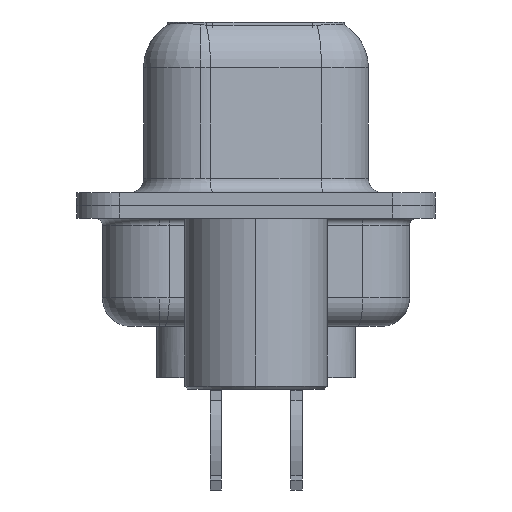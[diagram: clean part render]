
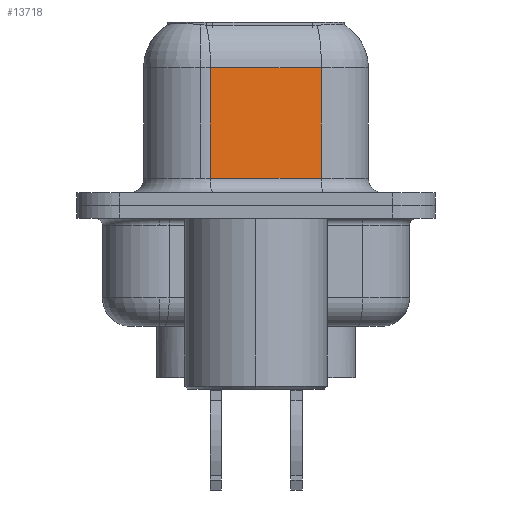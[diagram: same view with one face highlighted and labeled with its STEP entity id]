
A CAD part, left-side view. The second image highlights one B-rep face of the part: STEP entity #13718.
In plain terms, the highlighted planar face has unit normal (-0.985, -0.174, 0).
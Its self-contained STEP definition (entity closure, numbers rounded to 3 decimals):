
#380 = EDGE_CURVE ( 'NONE', #8218, #2512, #3110, .T. ) ;
#396 = CARTESIAN_POINT ( 'NONE',  ( 4.375, 1.603, 6.6 ) ) ;
#595 = DIRECTION ( 'NONE',  ( 0., 0., -1. ) ) ;
#1016 = VECTOR ( 'NONE', #13567, 1000. ) ;
#1240 = CARTESIAN_POINT ( 'NONE',  ( 5.063, -2.297, 6.6 ) ) ;
#1631 = LINE ( 'NONE', #396, #9218 ) ;
#1772 = DIRECTION ( 'NONE',  ( 0., 0., -1. ) ) ;
#2512 = VERTEX_POINT ( 'NONE', #15693 ) ;
#2651 = CARTESIAN_POINT ( 'NONE',  ( 5.063, -2.297, 4.85 ) ) ;
#3096 = DIRECTION ( 'NONE',  ( 0.985, 0.174, 0. ) ) ;
#3110 = LINE ( 'NONE', #4564, #11971 ) ;
#4564 = CARTESIAN_POINT ( 'NONE',  ( 5.063, -2.297, 6.6 ) ) ;
#5290 = LINE ( 'NONE', #16024, #9654 ) ;
#7243 = LINE ( 'NONE', #8904, #1016 ) ;
#8218 = VERTEX_POINT ( 'NONE', #2651 ) ;
#8488 = CARTESIAN_POINT ( 'NONE',  ( 4.375, 1.603, 0.95 ) ) ;
#8558 = VERTEX_POINT ( 'NONE', #8488 ) ;
#8904 = CARTESIAN_POINT ( 'NONE',  ( 5.063, -2.297, 4.85 ) ) ;
#9218 = VECTOR ( 'NONE', #595, 1000. ) ;
#9340 = EDGE_CURVE ( 'NONE', #17225, #8558, #1631, .T. ) ;
#9654 = VECTOR ( 'NONE', #11631, 1000. ) ;
#10092 = AXIS2_PLACEMENT_3D ( 'NONE', #1240, #3096, #15787 ) ;
#10482 = EDGE_LOOP ( 'NONE', ( #16739, #15724, #15220, #19773 ) ) ;
#11631 = DIRECTION ( 'NONE',  ( 0.174, -0.985, 0. ) ) ;
#11931 = CARTESIAN_POINT ( 'NONE',  ( 4.375, 1.603, 4.85 ) ) ;
#11971 = VECTOR ( 'NONE', #1772, 1000. ) ;
#13567 = DIRECTION ( 'NONE',  ( -0.174, 0.985, 0. ) ) ;
#13718 = ADVANCED_FACE ( 'NONE', ( #17352 ), #18724, .F. ) ;
#15220 = ORIENTED_EDGE ( 'NONE', *, *, #9340, .T. ) ;
#15693 = CARTESIAN_POINT ( 'NONE',  ( 5.063, -2.297, 0.95 ) ) ;
#15724 = ORIENTED_EDGE ( 'NONE', *, *, #19360, .T. ) ;
#15787 = DIRECTION ( 'NONE',  ( -0.174, 0.985, 0. ) ) ;
#16024 = CARTESIAN_POINT ( 'NONE',  ( 5.063, -2.297, 0.95 ) ) ;
#16739 = ORIENTED_EDGE ( 'NONE', *, *, #380, .F. ) ;
#17134 = EDGE_CURVE ( 'NONE', #8558, #2512, #5290, .T. ) ;
#17225 = VERTEX_POINT ( 'NONE', #11931 ) ;
#17352 = FACE_OUTER_BOUND ( 'NONE', #10482, .T. ) ;
#18724 = PLANE ( 'NONE',  #10092 ) ;
#19360 = EDGE_CURVE ( 'NONE', #8218, #17225, #7243, .T. ) ;
#19773 = ORIENTED_EDGE ( 'NONE', *, *, #17134, .T. ) ;
